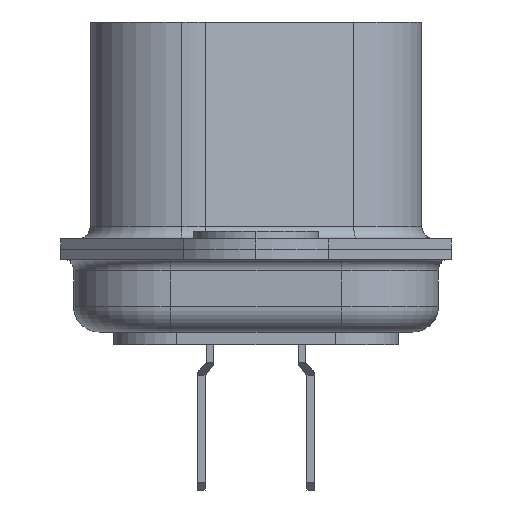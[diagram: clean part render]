
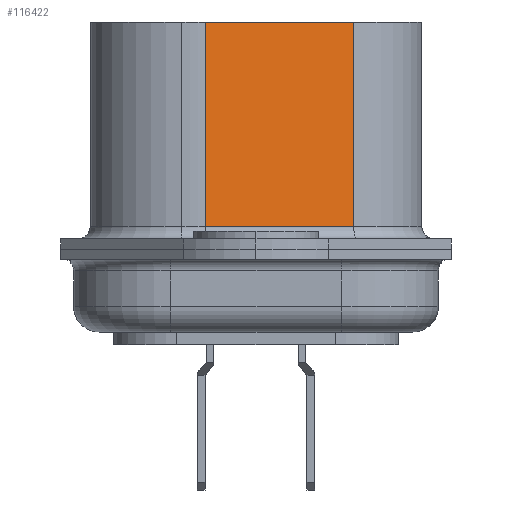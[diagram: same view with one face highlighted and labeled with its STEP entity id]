
A CAD part, left-side view. The second image highlights one B-rep face of the part: STEP entity #116422.
In plain terms, the highlighted planar face has unit normal (-0.966, -0.259, 0).
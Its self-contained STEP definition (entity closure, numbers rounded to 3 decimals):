
#3430 = PLANE ( 'NONE',  #25034 ) ;
#10932 = CARTESIAN_POINT ( 'NONE',  ( 6.467, -3.832, 9.3 ) ) ;
#15147 = VERTEX_POINT ( 'NONE', #131524 ) ;
#24971 = VECTOR ( 'NONE', #44436, 1000. ) ;
#25034 = AXIS2_PLACEMENT_3D ( 'NONE', #78082, #91438, #92199 ) ;
#31957 = VECTOR ( 'NONE', #32196, 1000. ) ;
#32196 = DIRECTION ( 'NONE',  ( 0., 0., -1. ) ) ;
#33046 = DIRECTION ( 'NONE',  ( 0.259, -0.966, 0. ) ) ;
#35467 = CARTESIAN_POINT ( 'NONE',  ( 6.467, -3.832, 9.3 ) ) ;
#40249 = EDGE_CURVE ( 'NONE', #15147, #99979, #58224, .T. ) ;
#41355 = CARTESIAN_POINT ( 'NONE',  ( 4.913, 1.968, 9.3 ) ) ;
#44436 = DIRECTION ( 'NONE',  ( 0., 0., -1. ) ) ;
#45583 = DIRECTION ( 'NONE',  ( 0.259, -0.966, 0. ) ) ;
#53082 = EDGE_CURVE ( 'NONE', #127159, #139470, #141516, .T. ) ;
#58224 = LINE ( 'NONE', #141588, #114397 ) ;
#60556 = ORIENTED_EDGE ( 'NONE', *, *, #40249, .T. ) ;
#66398 = ORIENTED_EDGE ( 'NONE', *, *, #147518, .T. ) ;
#68014 = LINE ( 'NONE', #41355, #24971 ) ;
#72348 = EDGE_LOOP ( 'NONE', ( #66398, #60556, #102259, #93148 ) ) ;
#76114 = VECTOR ( 'NONE', #45583, 1000. ) ;
#78082 = CARTESIAN_POINT ( 'NONE',  ( 6.467, -3.832, 9.3 ) ) ;
#78611 = CARTESIAN_POINT ( 'NONE',  ( 4.913, 1.968, 9.3 ) ) ;
#91438 = DIRECTION ( 'NONE',  ( 0.966, 0.259, 0. ) ) ;
#92199 = DIRECTION ( 'NONE',  ( -0.259, 0.966, 0. ) ) ;
#93148 = ORIENTED_EDGE ( 'NONE', *, *, #53082, .F. ) ;
#95058 = LINE ( 'NONE', #10932, #31957 ) ;
#98303 = CARTESIAN_POINT ( 'NONE',  ( 6.467, -3.832, 1.3 ) ) ;
#99979 = VERTEX_POINT ( 'NONE', #98303 ) ;
#102259 = ORIENTED_EDGE ( 'NONE', *, *, #144479, .F. ) ;
#111190 = FACE_OUTER_BOUND ( 'NONE', #72348, .T. ) ;
#114397 = VECTOR ( 'NONE', #33046, 1000. ) ;
#116422 = ADVANCED_FACE ( 'NONE', ( #111190 ), #3430, .F. ) ;
#127159 = VERTEX_POINT ( 'NONE', #78611 ) ;
#131245 = CARTESIAN_POINT ( 'NONE',  ( 6.467, -3.832, 9.3 ) ) ;
#131524 = CARTESIAN_POINT ( 'NONE',  ( 4.913, 1.968, 1.3 ) ) ;
#139470 = VERTEX_POINT ( 'NONE', #35467 ) ;
#141516 = LINE ( 'NONE', #131245, #76114 ) ;
#141588 = CARTESIAN_POINT ( 'NONE',  ( 6.467, -3.832, 1.3 ) ) ;
#144479 = EDGE_CURVE ( 'NONE', #139470, #99979, #95058, .T. ) ;
#147518 = EDGE_CURVE ( 'NONE', #127159, #15147, #68014, .T. ) ;
